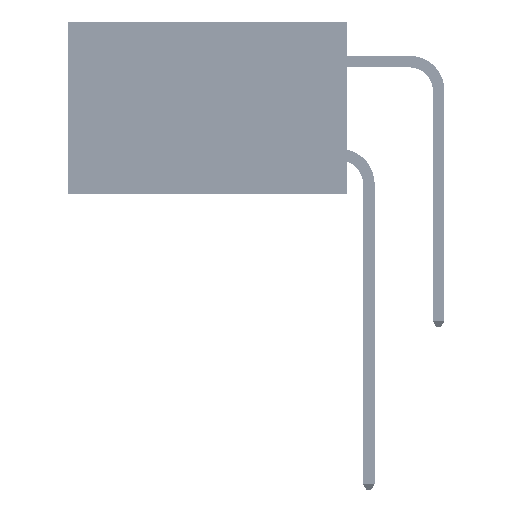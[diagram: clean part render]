
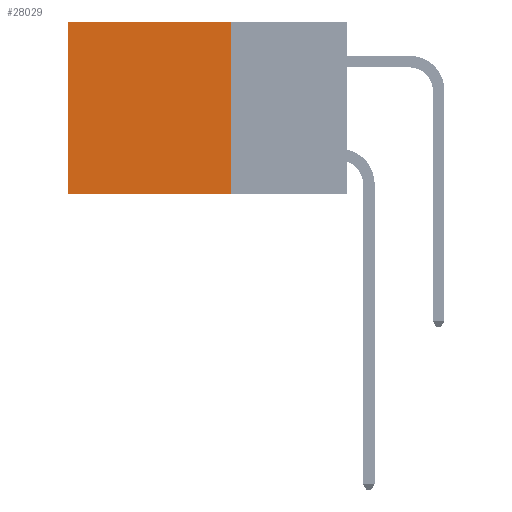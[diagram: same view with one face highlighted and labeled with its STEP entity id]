
A CAD part, left-side view. The second image highlights one B-rep face of the part: STEP entity #28029.
In plain terms, the highlighted planar face has unit normal (-1, 0, 0).
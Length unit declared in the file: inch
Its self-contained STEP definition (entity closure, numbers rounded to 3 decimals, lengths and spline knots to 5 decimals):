
#120 = PLANE ( 'NONE',  #17958 ) ;
#559 = ORIENTED_EDGE ( 'NONE', *, *, #26795, .T. ) ;
#1015 = CARTESIAN_POINT ( 'NONE',  ( 0.2875, 0.25, 0. ) ) ;
#1793 = DIRECTION ( 'NONE',  ( 0., 1., 0. ) ) ;
#4109 = CARTESIAN_POINT ( 'NONE',  ( 0.2875, 0.25, -0.37 ) ) ;
#4583 = EDGE_CURVE ( 'NONE', #11133, #36062, #22779, .T. ) ;
#7639 = DIRECTION ( 'NONE',  ( 0., 0., -1. ) ) ;
#9482 = EDGE_CURVE ( 'NONE', #36062, #10613, #39581, .T. ) ;
#10613 = VERTEX_POINT ( 'NONE', #42588 ) ;
#11133 = VERTEX_POINT ( 'NONE', #1015 ) ;
#13517 = VECTOR ( 'NONE', #45367, 39.37008 ) ;
#15536 = VECTOR ( 'NONE', #37505, 39.37008 ) ;
#17958 = AXIS2_PLACEMENT_3D ( 'NONE', #37391, #46136, #7639 ) ;
#18509 = CARTESIAN_POINT ( 'NONE',  ( 0.2875, 0.25, 0. ) ) ;
#18832 = CARTESIAN_POINT ( 'NONE',  ( 0.2875, 0.6, 0. ) ) ;
#20794 = CARTESIAN_POINT ( 'NONE',  ( 0.2875, 0.6, 0. ) ) ;
#22779 = LINE ( 'NONE', #18509, #15536 ) ;
#23848 = VECTOR ( 'NONE', #1793, 39.37008 ) ;
#26795 = EDGE_CURVE ( 'NONE', #49141, #10613, #38072, .T. ) ;
#28029 = ADVANCED_FACE ( 'NONE', ( #30898 ), #120, .F. ) ;
#28953 = ORIENTED_EDGE ( 'NONE', *, *, #4583, .F. ) ;
#29443 = ORIENTED_EDGE ( 'NONE', *, *, #41518, .T. ) ;
#30141 = LINE ( 'NONE', #48615, #13517 ) ;
#30898 = FACE_OUTER_BOUND ( 'NONE', #35536, .T. ) ;
#35160 = ORIENTED_EDGE ( 'NONE', *, *, #9482, .F. ) ;
#35536 = EDGE_LOOP ( 'NONE', ( #559, #35160, #28953, #29443 ) ) ;
#36062 = VERTEX_POINT ( 'NONE', #4109 ) ;
#37391 = CARTESIAN_POINT ( 'NONE',  ( 0.2875, 0.25, 0. ) ) ;
#37505 = DIRECTION ( 'NONE',  ( 0., 0., -1. ) ) ;
#38072 = LINE ( 'NONE', #18832, #47312 ) ;
#39581 = LINE ( 'NONE', #43564, #23848 ) ;
#41518 = EDGE_CURVE ( 'NONE', #11133, #49141, #30141, .T. ) ;
#42588 = CARTESIAN_POINT ( 'NONE',  ( 0.2875, 0.6, -0.37 ) ) ;
#42839 = DIRECTION ( 'NONE',  ( 0., 0., -1. ) ) ;
#43564 = CARTESIAN_POINT ( 'NONE',  ( 0.2875, 0.25, -0.37 ) ) ;
#45367 = DIRECTION ( 'NONE',  ( 0., 1., 0. ) ) ;
#46136 = DIRECTION ( 'NONE',  ( 1., 0., 0. ) ) ;
#47312 = VECTOR ( 'NONE', #42839, 39.37008 ) ;
#48615 = CARTESIAN_POINT ( 'NONE',  ( 0.2875, 0.25, 0. ) ) ;
#49141 = VERTEX_POINT ( 'NONE', #20794 ) ;
